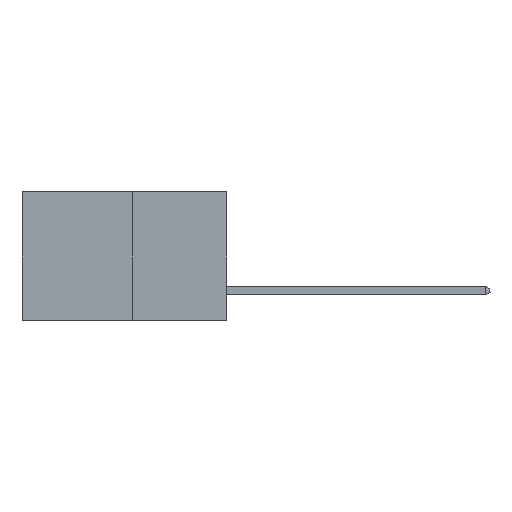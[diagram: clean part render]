
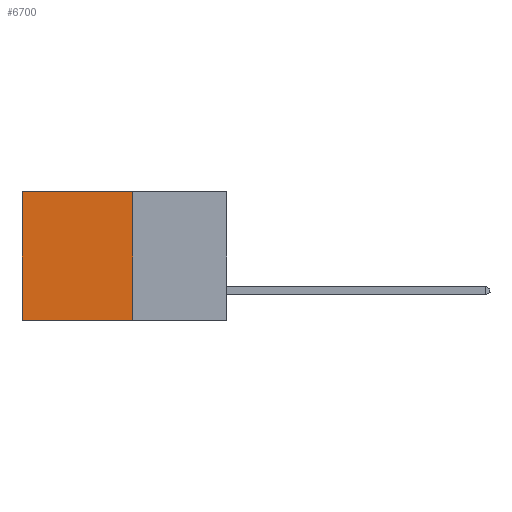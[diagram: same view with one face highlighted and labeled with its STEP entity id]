
A CAD part, left-side view. The second image highlights one B-rep face of the part: STEP entity #6700.
In plain terms, the highlighted planar face has unit normal (-1, 0, 0).
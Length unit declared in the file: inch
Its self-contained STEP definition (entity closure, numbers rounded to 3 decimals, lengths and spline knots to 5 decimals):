
#265 = ORIENTED_EDGE ( 'NONE', *, *, #15614, .F. ) ;
#889 = LINE ( 'NONE', #4949, #10728 ) ;
#1372 = CARTESIAN_POINT ( 'NONE',  ( 0.277, 0.27, -0.37 ) ) ;
#1412 = ORIENTED_EDGE ( 'NONE', *, *, #2484, .T. ) ;
#1737 = CARTESIAN_POINT ( 'NONE',  ( 0.277, 0.59, -0.37 ) ) ;
#2448 = VERTEX_POINT ( 'NONE', #14557 ) ;
#2484 = EDGE_CURVE ( 'NONE', #14219, #2448, #4866, .T. ) ;
#2819 = ORIENTED_EDGE ( 'NONE', *, *, #5115, .T. ) ;
#4866 = LINE ( 'NONE', #15766, #14229 ) ;
#4949 = CARTESIAN_POINT ( 'NONE',  ( 0.277, 0.27, -0.37 ) ) ;
#5035 = VERTEX_POINT ( 'NONE', #5589 ) ;
#5115 = EDGE_CURVE ( 'NONE', #2448, #5035, #5754, .T. ) ;
#5589 = CARTESIAN_POINT ( 'NONE',  ( 0.277, 0.59, -0.37 ) ) ;
#5754 = LINE ( 'NONE', #1737, #11805 ) ;
#6191 = DIRECTION ( 'NONE',  ( 0., 1., 0. ) ) ;
#6428 = EDGE_LOOP ( 'NONE', ( #2819, #265, #13371, #1412 ) ) ;
#6700 = ADVANCED_FACE ( 'NONE', ( #13916 ), #10366, .F. ) ;
#7301 = CARTESIAN_POINT ( 'NONE',  ( 0.277, 0.27, -0.37 ) ) ;
#8574 = VERTEX_POINT ( 'NONE', #1372 ) ;
#9558 = EDGE_CURVE ( 'NONE', #14219, #8574, #15339, .T. ) ;
#10366 = PLANE ( 'NONE',  #13849 ) ;
#10446 = DIRECTION ( 'NONE',  ( 0., 0., -1. ) ) ;
#10590 = DIRECTION ( 'NONE',  ( 1., 0., 0. ) ) ;
#10728 = VECTOR ( 'NONE', #6191, 39.37008 ) ;
#10750 = CARTESIAN_POINT ( 'NONE',  ( 0.277, 0.27, -0.37 ) ) ;
#11805 = VECTOR ( 'NONE', #11819, 39.37008 ) ;
#11819 = DIRECTION ( 'NONE',  ( 0., 0., -1. ) ) ;
#11987 = CARTESIAN_POINT ( 'NONE',  ( 0.277, 0.27, 0. ) ) ;
#12582 = DIRECTION ( 'NONE',  ( 0., 1., 0. ) ) ;
#13371 = ORIENTED_EDGE ( 'NONE', *, *, #9558, .F. ) ;
#13849 = AXIS2_PLACEMENT_3D ( 'NONE', #10750, #10590, #10446 ) ;
#13916 = FACE_OUTER_BOUND ( 'NONE', #6428, .T. ) ;
#14219 = VERTEX_POINT ( 'NONE', #11987 ) ;
#14229 = VECTOR ( 'NONE', #12582, 39.37008 ) ;
#14557 = CARTESIAN_POINT ( 'NONE',  ( 0.277, 0.59, 0. ) ) ;
#14595 = DIRECTION ( 'NONE',  ( 0., 0., -1. ) ) ;
#14953 = VECTOR ( 'NONE', #14595, 39.37008 ) ;
#15339 = LINE ( 'NONE', #7301, #14953 ) ;
#15614 = EDGE_CURVE ( 'NONE', #8574, #5035, #889, .T. ) ;
#15766 = CARTESIAN_POINT ( 'NONE',  ( 0.277, 0.27, 0. ) ) ;
